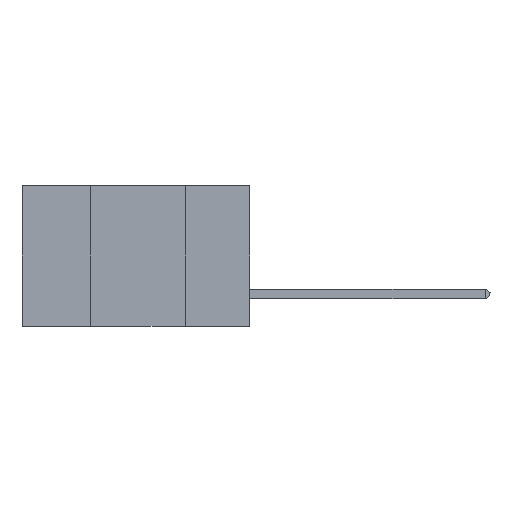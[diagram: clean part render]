
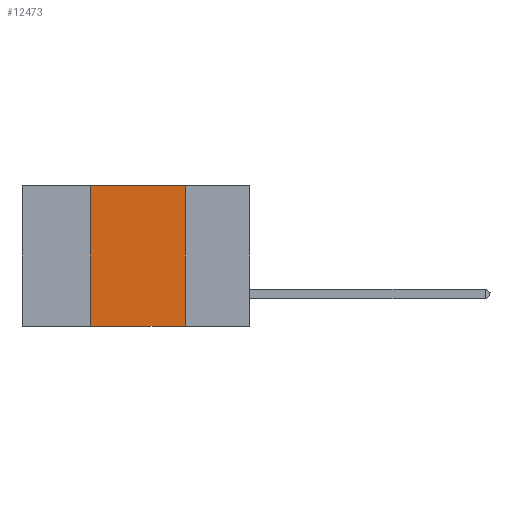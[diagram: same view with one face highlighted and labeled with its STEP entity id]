
A CAD part, left-side view. The second image highlights one B-rep face of the part: STEP entity #12473.
In plain terms, the highlighted planar face has unit normal (-1, 0, 0).
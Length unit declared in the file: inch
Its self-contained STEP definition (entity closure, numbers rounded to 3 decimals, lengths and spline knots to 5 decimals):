
#756 = DIRECTION ( 'NONE',  ( 0., 0., 1. ) ) ;
#854 = DIRECTION ( 'NONE',  ( 0., -1., 0. ) ) ;
#975 = VERTEX_POINT ( 'NONE', #10277 ) ;
#1147 = DIRECTION ( 'NONE',  ( 1., 0., 0. ) ) ;
#1469 = CARTESIAN_POINT ( 'NONE',  ( 0., 0.17, -0.37 ) ) ;
#1580 = DIRECTION ( 'NONE',  ( 0., -1., 0. ) ) ;
#1631 = DIRECTION ( 'NONE',  ( 0., 0., -1. ) ) ;
#2450 = VECTOR ( 'NONE', #854, 39.37008 ) ;
#2681 = VERTEX_POINT ( 'NONE', #7640 ) ;
#2853 = CARTESIAN_POINT ( 'NONE',  ( 0., 0.6, -0.37 ) ) ;
#3192 = LINE ( 'NONE', #6707, #7210 ) ;
#3424 = CARTESIAN_POINT ( 'NONE',  ( 0., 0.17, 0. ) ) ;
#3495 = DIRECTION ( 'NONE',  ( 0., 0., -1. ) ) ;
#3925 = VERTEX_POINT ( 'NONE', #1469 ) ;
#3951 = EDGE_CURVE ( 'NONE', #9628, #3925, #11539, .T. ) ;
#3956 = LINE ( 'NONE', #2853, #2450 ) ;
#4355 = PLANE ( 'NONE',  #5058 ) ;
#4448 = EDGE_CURVE ( 'NONE', #975, #9628, #3192, .T. ) ;
#4602 = EDGE_LOOP ( 'NONE', ( #12873, #8441, #11283, #13696 ) ) ;
#4794 = VECTOR ( 'NONE', #756, 39.37008 ) ;
#5058 = AXIS2_PLACEMENT_3D ( 'NONE', #6484, #1147, #1631 ) ;
#6484 = CARTESIAN_POINT ( 'NONE',  ( 0., 0.6, 0. ) ) ;
#6658 = LINE ( 'NONE', #7065, #4794 ) ;
#6707 = CARTESIAN_POINT ( 'NONE',  ( 0., 0.6, 0. ) ) ;
#7065 = CARTESIAN_POINT ( 'NONE',  ( 0., 0.42, 0. ) ) ;
#7210 = VECTOR ( 'NONE', #1580, 39.37008 ) ;
#7530 = CARTESIAN_POINT ( 'NONE',  ( 0., 0.17, 0. ) ) ;
#7640 = CARTESIAN_POINT ( 'NONE',  ( 0., 0.42, -0.37 ) ) ;
#8441 = ORIENTED_EDGE ( 'NONE', *, *, #4448, .F. ) ;
#9483 = FACE_OUTER_BOUND ( 'NONE', #4602, .T. ) ;
#9628 = VERTEX_POINT ( 'NONE', #3424 ) ;
#10199 = VECTOR ( 'NONE', #3495, 39.37008 ) ;
#10277 = CARTESIAN_POINT ( 'NONE',  ( 0., 0.42, 0. ) ) ;
#11283 = ORIENTED_EDGE ( 'NONE', *, *, #11815, .F. ) ;
#11539 = LINE ( 'NONE', #7530, #10199 ) ;
#11815 = EDGE_CURVE ( 'NONE', #2681, #975, #6658, .T. ) ;
#12426 = EDGE_CURVE ( 'NONE', #2681, #3925, #3956, .T. ) ;
#12473 = ADVANCED_FACE ( 'NONE', ( #9483 ), #4355, .F. ) ;
#12873 = ORIENTED_EDGE ( 'NONE', *, *, #3951, .F. ) ;
#13696 = ORIENTED_EDGE ( 'NONE', *, *, #12426, .T. ) ;
